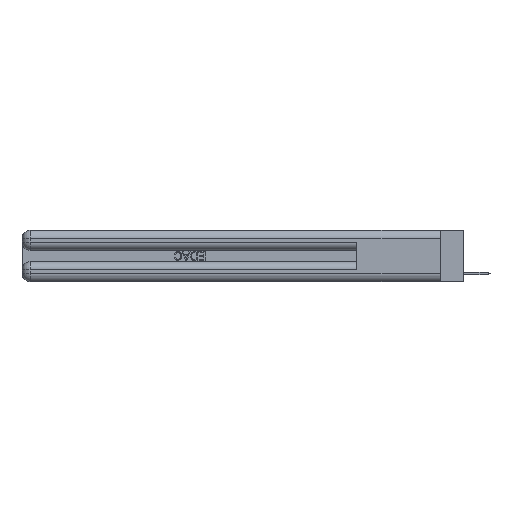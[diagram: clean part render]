
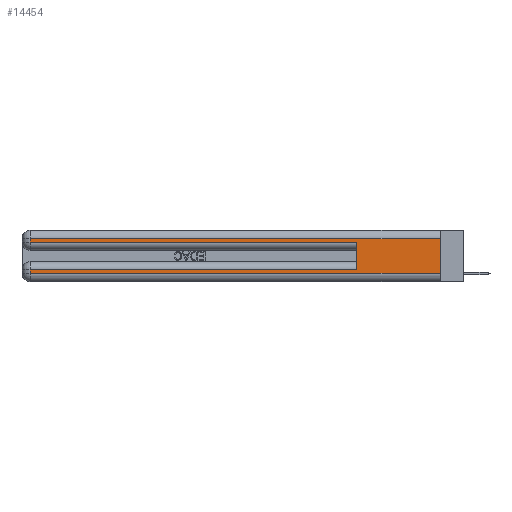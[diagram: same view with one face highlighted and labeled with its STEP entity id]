
A CAD part, left-side view. The second image highlights one B-rep face of the part: STEP entity #14454.
In plain terms, the highlighted planar face has unit normal (-1, 0, 0).
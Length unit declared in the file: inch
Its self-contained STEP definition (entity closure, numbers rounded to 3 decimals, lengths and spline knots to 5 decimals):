
#223 = CARTESIAN_POINT ( 'NONE',  ( 0., 0., 0.31 ) ) ;
#422 = CARTESIAN_POINT ( 'NONE',  ( 0., 0., 0.31 ) ) ;
#534 = EDGE_CURVE ( 'NONE', #5057, #22898, #18284, .T. ) ;
#1347 = DIRECTION ( 'NONE',  ( 0., 0., -1. ) ) ;
#1737 = LINE ( 'NONE', #223, #27338 ) ;
#2152 = DIRECTION ( 'NONE',  ( 0., 0., -1. ) ) ;
#2896 = VERTEX_POINT ( 'NONE', #422 ) ;
#3248 = LINE ( 'NONE', #12562, #12062 ) ;
#4451 = LINE ( 'NONE', #24876, #7260 ) ;
#5034 = FACE_OUTER_BOUND ( 'NONE', #29023, .T. ) ;
#5057 = VERTEX_POINT ( 'NONE', #21572 ) ;
#5135 = VECTOR ( 'NONE', #9594, 39.37008 ) ;
#5798 = VERTEX_POINT ( 'NONE', #6973 ) ;
#6973 = CARTESIAN_POINT ( 'NONE',  ( 0., 2.94, 0.31 ) ) ;
#7260 = VECTOR ( 'NONE', #13719, 39.37008 ) ;
#8172 = DIRECTION ( 'NONE',  ( 1., 0., 0. ) ) ;
#8383 = EDGE_CURVE ( 'NONE', #2896, #5798, #1737, .T. ) ;
#8439 = ORIENTED_EDGE ( 'NONE', *, *, #534, .T. ) ;
#8636 = VERTEX_POINT ( 'NONE', #12674 ) ;
#9021 = LINE ( 'NONE', #20985, #5135 ) ;
#9240 = EDGE_CURVE ( 'NONE', #5798, #25446, #4451, .T. ) ;
#9268 = CARTESIAN_POINT ( 'NONE',  ( 0., 0., 0.37 ) ) ;
#9594 = DIRECTION ( 'NONE',  ( 0., 0., 1. ) ) ;
#10244 = CARTESIAN_POINT ( 'NONE',  ( 0., 2.94, 0.085 ) ) ;
#10629 = DIRECTION ( 'NONE',  ( 0., -1., 0. ) ) ;
#12002 = EDGE_CURVE ( 'NONE', #27497, #8636, #9021, .T. ) ;
#12062 = VECTOR ( 'NONE', #28323, 39.37008 ) ;
#12227 = CARTESIAN_POINT ( 'NONE',  ( 0., 0., 0.06 ) ) ;
#12344 = VECTOR ( 'NONE', #25699, 39.37008 ) ;
#12444 = VECTOR ( 'NONE', #15999, 39.37008 ) ;
#12562 = CARTESIAN_POINT ( 'NONE',  ( 0., 0., 0.085 ) ) ;
#12617 = CARTESIAN_POINT ( 'NONE',  ( 0., 0., 0.285 ) ) ;
#12674 = CARTESIAN_POINT ( 'NONE',  ( 0., 0.6, 0.285 ) ) ;
#12746 = ORIENTED_EDGE ( 'NONE', *, *, #8383, .T. ) ;
#13719 = DIRECTION ( 'NONE',  ( 0., 0., -1. ) ) ;
#14189 = EDGE_CURVE ( 'NONE', #2896, #22898, #21528, .T. ) ;
#14454 = ADVANCED_FACE ( 'NONE', ( #5034 ), #19197, .F. ) ;
#14818 = EDGE_CURVE ( 'NONE', #27497, #15411, #3248, .T. ) ;
#15212 = ORIENTED_EDGE ( 'NONE', *, *, #14189, .F. ) ;
#15368 = ORIENTED_EDGE ( 'NONE', *, *, #15521, .T. ) ;
#15411 = VERTEX_POINT ( 'NONE', #10244 ) ;
#15521 = EDGE_CURVE ( 'NONE', #25446, #8636, #27413, .T. ) ;
#15999 = DIRECTION ( 'NONE',  ( 0., 0., -1. ) ) ;
#16231 = VECTOR ( 'NONE', #10629, 39.37008 ) ;
#17409 = CARTESIAN_POINT ( 'NONE',  ( 0., 0., 0.06 ) ) ;
#18284 = LINE ( 'NONE', #12227, #12344 ) ;
#19197 = PLANE ( 'NONE',  #27081 ) ;
#20627 = ORIENTED_EDGE ( 'NONE', *, *, #27461, .T. ) ;
#20985 = CARTESIAN_POINT ( 'NONE',  ( 0., 0.6, 0.145 ) ) ;
#21429 = CARTESIAN_POINT ( 'NONE',  ( 0., 0., 0.37 ) ) ;
#21528 = LINE ( 'NONE', #9268, #12444 ) ;
#21572 = CARTESIAN_POINT ( 'NONE',  ( 0., 2.94, 0.06 ) ) ;
#22182 = DIRECTION ( 'NONE',  ( 0., 1., 0. ) ) ;
#22350 = CARTESIAN_POINT ( 'NONE',  ( 0., 0.6, 0.085 ) ) ;
#22898 = VERTEX_POINT ( 'NONE', #17409 ) ;
#23785 = ORIENTED_EDGE ( 'NONE', *, *, #14818, .T. ) ;
#24048 = VECTOR ( 'NONE', #2152, 39.37008 ) ;
#24332 = ORIENTED_EDGE ( 'NONE', *, *, #12002, .F. ) ;
#24876 = CARTESIAN_POINT ( 'NONE',  ( 0., 2.94, 0.37 ) ) ;
#25446 = VERTEX_POINT ( 'NONE', #26636 ) ;
#25454 = LINE ( 'NONE', #29053, #24048 ) ;
#25699 = DIRECTION ( 'NONE',  ( 0., -1., 0. ) ) ;
#25887 = ORIENTED_EDGE ( 'NONE', *, *, #9240, .T. ) ;
#26636 = CARTESIAN_POINT ( 'NONE',  ( 0., 2.94, 0.285 ) ) ;
#27081 = AXIS2_PLACEMENT_3D ( 'NONE', #21429, #8172, #1347 ) ;
#27338 = VECTOR ( 'NONE', #22182, 39.37008 ) ;
#27413 = LINE ( 'NONE', #12617, #16231 ) ;
#27461 = EDGE_CURVE ( 'NONE', #15411, #5057, #25454, .T. ) ;
#27497 = VERTEX_POINT ( 'NONE', #22350 ) ;
#28323 = DIRECTION ( 'NONE',  ( 0., 1., 0. ) ) ;
#29023 = EDGE_LOOP ( 'NONE', ( #15212, #12746, #25887, #15368, #24332, #23785, #20627, #8439 ) ) ;
#29053 = CARTESIAN_POINT ( 'NONE',  ( 0., 2.94, 0.37 ) ) ;
